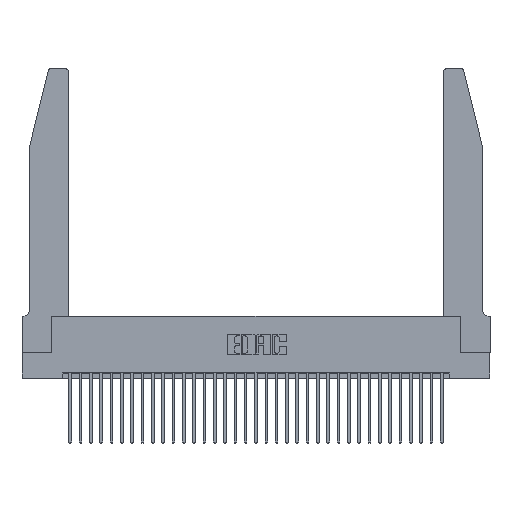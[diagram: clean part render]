
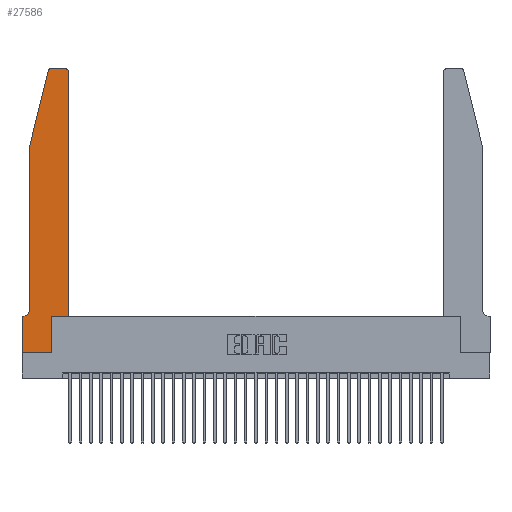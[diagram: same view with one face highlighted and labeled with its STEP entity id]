
A CAD part, top view. The second image highlights one B-rep face of the part: STEP entity #27586.
In plain terms, the highlighted planar face has unit normal (0, 0, 1).
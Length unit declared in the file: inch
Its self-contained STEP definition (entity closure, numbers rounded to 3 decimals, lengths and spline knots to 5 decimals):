
#1044 = LINE ( 'NONE', #24353, #5614 ) ;
#1261 = AXIS2_PLACEMENT_3D ( 'NONE', #30730, #17402, #17047 ) ;
#1269 = LINE ( 'NONE', #11646, #28844 ) ;
#1774 = VERTEX_POINT ( 'NONE', #23966 ) ;
#2354 = VECTOR ( 'NONE', #22822, 39.37008 ) ;
#2534 = DIRECTION ( 'NONE',  ( 0., 0., -1. ) ) ;
#2991 = VERTEX_POINT ( 'NONE', #21759 ) ;
#4453 = DIRECTION ( 'NONE',  ( 0., 0., 1. ) ) ;
#4657 = AXIS2_PLACEMENT_3D ( 'NONE', #31437, #2534, #13066 ) ;
#4948 = VERTEX_POINT ( 'NONE', #28981 ) ;
#5371 = ORIENTED_EDGE ( 'NONE', *, *, #18641, .T. ) ;
#5396 = ORIENTED_EDGE ( 'NONE', *, *, #10358, .T. ) ;
#5495 = VERTEX_POINT ( 'NONE', #25967 ) ;
#5523 = CARTESIAN_POINT ( 'NONE',  ( 0.2865, 0.35, 0.37 ) ) ;
#5581 = ORIENTED_EDGE ( 'NONE', *, *, #32801, .T. ) ;
#5614 = VECTOR ( 'NONE', #13857, 39.37008 ) ;
#5750 = EDGE_CURVE ( 'NONE', #34244, #27539, #1044, .T. ) ;
#6007 = CARTESIAN_POINT ( 'NONE',  ( 0., 0.35, 0.37 ) ) ;
#6024 = DIRECTION ( 'NONE',  ( -1., 0., 0. ) ) ;
#6217 = DIRECTION ( 'NONE',  ( -1., 0., 0. ) ) ;
#6997 = CIRCLE ( 'NONE', #18009, 0.03 ) ;
#7269 = LINE ( 'NONE', #21630, #29381 ) ;
#7434 = DIRECTION ( 'NONE',  ( 1., 0., 0. ) ) ;
#7469 = ORIENTED_EDGE ( 'NONE', *, *, #24453, .T. ) ;
#7637 = VERTEX_POINT ( 'NONE', #9585 ) ;
#7766 = VERTEX_POINT ( 'NONE', #24778 ) ;
#7916 = DIRECTION ( 'NONE',  ( 0., -1., 0. ) ) ;
#8267 = CARTESIAN_POINT ( 'NONE',  ( 0.284, 2.75, 0.37 ) ) ;
#8309 = DIRECTION ( 'NONE',  ( 0., 1., 0. ) ) ;
#8636 = VECTOR ( 'NONE', #8309, 39.37008 ) ;
#9374 = LINE ( 'NONE', #9768, #2354 ) ;
#9443 = CARTESIAN_POINT ( 'NONE',  ( 0., 0.35, 0.37 ) ) ;
#9585 = CARTESIAN_POINT ( 'NONE',  ( 0.0755, 0.42, 0.37 ) ) ;
#9603 = ORIENTED_EDGE ( 'NONE', *, *, #20133, .T. ) ;
#9768 = CARTESIAN_POINT ( 'NONE',  ( 0.0755, 2., 0.37 ) ) ;
#10036 = LINE ( 'NONE', #27269, #33852 ) ;
#10358 = EDGE_CURVE ( 'NONE', #2991, #1774, #9374, .T. ) ;
#10727 = VERTEX_POINT ( 'NONE', #22893 ) ;
#10766 = VERTEX_POINT ( 'NONE', #24979 ) ;
#11066 = LINE ( 'NONE', #15331, #33251 ) ;
#11196 = VERTEX_POINT ( 'NONE', #31614 ) ;
#11646 = CARTESIAN_POINT ( 'NONE',  ( 0.2605, 2.75, 0.37 ) ) ;
#11811 = CARTESIAN_POINT ( 'NONE',  ( 0.4505, 0.35, 0.37 ) ) ;
#12561 = LINE ( 'NONE', #11811, #13008 ) ;
#13008 = VECTOR ( 'NONE', #30892, 39.37008 ) ;
#13066 = DIRECTION ( 'NONE',  ( -1., 0., 0. ) ) ;
#13088 = FACE_OUTER_BOUND ( 'NONE', #23824, .T. ) ;
#13345 = DIRECTION ( 'NONE',  ( 1., 0., 0. ) ) ;
#13494 = EDGE_CURVE ( 'NONE', #17254, #2991, #16128, .T. ) ;
#13581 = ORIENTED_EDGE ( 'NONE', *, *, #22711, .T. ) ;
#13830 = LINE ( 'NONE', #31741, #28941 ) ;
#13857 = DIRECTION ( 'NONE',  ( 0., -1., 0. ) ) ;
#14133 = CIRCLE ( 'NONE', #4657, 0.07 ) ;
#15331 = CARTESIAN_POINT ( 'NONE',  ( 0., 0., 0.37 ) ) ;
#15649 = ORIENTED_EDGE ( 'NONE', *, *, #23560, .T. ) ;
#16122 = EDGE_CURVE ( 'NONE', #11196, #5495, #21562, .T. ) ;
#16128 = CIRCLE ( 'NONE', #1261, 0.03 ) ;
#17047 = DIRECTION ( 'NONE',  ( 1., 0., 0. ) ) ;
#17254 = VERTEX_POINT ( 'NONE', #8267 ) ;
#17365 = DIRECTION ( 'NONE',  ( 1., 0., 0. ) ) ;
#17402 = DIRECTION ( 'NONE',  ( 0., 0., 1. ) ) ;
#18009 = AXIS2_PLACEMENT_3D ( 'NONE', #18811, #24067, #13345 ) ;
#18641 = EDGE_CURVE ( 'NONE', #4948, #17254, #1269, .T. ) ;
#18811 = CARTESIAN_POINT ( 'NONE',  ( 0.4205, 2.72, 0.37 ) ) ;
#19172 = DIRECTION ( 'NONE',  ( 1., 0., 0. ) ) ;
#20133 = EDGE_CURVE ( 'NONE', #10727, #10766, #12561, .T. ) ;
#20863 = ORIENTED_EDGE ( 'NONE', *, *, #13494, .T. ) ;
#21562 = LINE ( 'NONE', #5523, #8636 ) ;
#21630 = CARTESIAN_POINT ( 'NONE',  ( 0.4505, 0.35, 0.37 ) ) ;
#21759 = CARTESIAN_POINT ( 'NONE',  ( 0.25487, 2.72718, 0.37 ) ) ;
#22711 = EDGE_CURVE ( 'NONE', #10766, #4948, #6997, .T. ) ;
#22822 = DIRECTION ( 'NONE',  ( -0.239, -0.971, 0. ) ) ;
#22893 = CARTESIAN_POINT ( 'NONE',  ( 0.4505, 0.35, 0.37 ) ) ;
#23560 = EDGE_CURVE ( 'NONE', #7766, #34244, #10036, .T. ) ;
#23824 = EDGE_LOOP ( 'NONE', ( #5371, #20863, #5396, #28962, #7469, #15649, #26749, #25791, #33625, #5581, #9603, #13581 ) ) ;
#23966 = CARTESIAN_POINT ( 'NONE',  ( 0.0755, 2., 0.37 ) ) ;
#24067 = DIRECTION ( 'NONE',  ( 0., 0., 1. ) ) ;
#24353 = CARTESIAN_POINT ( 'NONE',  ( 0., 0., 0.37 ) ) ;
#24453 = EDGE_CURVE ( 'NONE', #7637, #7766, #14133, .T. ) ;
#24778 = CARTESIAN_POINT ( 'NONE',  ( 0.0055, 0.35, 0.37 ) ) ;
#24979 = CARTESIAN_POINT ( 'NONE',  ( 0.4505, 2.72, 0.37 ) ) ;
#25372 = CARTESIAN_POINT ( 'NONE',  ( 0., 0., 0.37 ) ) ;
#25663 = PLANE ( 'NONE',  #31990 ) ;
#25791 = ORIENTED_EDGE ( 'NONE', *, *, #31291, .T. ) ;
#25967 = CARTESIAN_POINT ( 'NONE',  ( 0.2865, 0.35, 0.37 ) ) ;
#26749 = ORIENTED_EDGE ( 'NONE', *, *, #5750, .T. ) ;
#27269 = CARTESIAN_POINT ( 'NONE',  ( 0.0755, 0.35, 0.37 ) ) ;
#27539 = VERTEX_POINT ( 'NONE', #25372 ) ;
#27586 = ADVANCED_FACE ( 'NONE', ( #13088 ), #25663, .T. ) ;
#28844 = VECTOR ( 'NONE', #6217, 39.37008 ) ;
#28941 = VECTOR ( 'NONE', #7916, 39.37008 ) ;
#28962 = ORIENTED_EDGE ( 'NONE', *, *, #33984, .T. ) ;
#28981 = CARTESIAN_POINT ( 'NONE',  ( 0.4205, 2.75, 0.37 ) ) ;
#29381 = VECTOR ( 'NONE', #19172, 39.37008 ) ;
#30730 = CARTESIAN_POINT ( 'NONE',  ( 0.284, 2.72, 0.37 ) ) ;
#30892 = DIRECTION ( 'NONE',  ( 0., 1., 0. ) ) ;
#31291 = EDGE_CURVE ( 'NONE', #27539, #11196, #11066, .T. ) ;
#31437 = CARTESIAN_POINT ( 'NONE',  ( 0.0055, 0.42, 0.37 ) ) ;
#31614 = CARTESIAN_POINT ( 'NONE',  ( 0.2865, 0., 0.37 ) ) ;
#31741 = CARTESIAN_POINT ( 'NONE',  ( 0.0755, 2., 0.37 ) ) ;
#31990 = AXIS2_PLACEMENT_3D ( 'NONE', #9443, #4453, #17365 ) ;
#32801 = EDGE_CURVE ( 'NONE', #5495, #10727, #7269, .T. ) ;
#33251 = VECTOR ( 'NONE', #7434, 39.37008 ) ;
#33625 = ORIENTED_EDGE ( 'NONE', *, *, #16122, .T. ) ;
#33852 = VECTOR ( 'NONE', #6024, 39.37008 ) ;
#33984 = EDGE_CURVE ( 'NONE', #1774, #7637, #13830, .T. ) ;
#34244 = VERTEX_POINT ( 'NONE', #6007 ) ;
